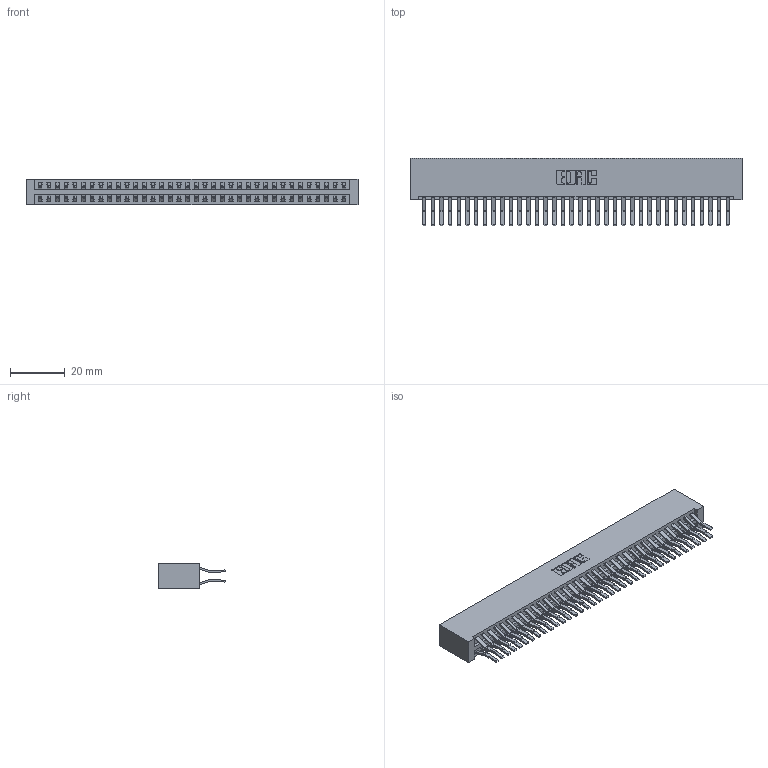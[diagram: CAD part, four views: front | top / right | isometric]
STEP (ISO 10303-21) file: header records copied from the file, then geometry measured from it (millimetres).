
FILE_DESCRIPTION (( 'STEP AP203' ), '1' );
FILE_NAME ('396-072-560-201.STEP', '2018-09-09T11:05:24', ( '' ), ( '' ), 'SwSTEP 2.0', 'SolidWorks 2016', '' );
FILE_SCHEMA (( 'CONFIG_CONTROL_DESIGN' ));
Length unit declared in the file: inch
Products named in the file (3): 346 Part_No Mounting Lugs; 345-292-001_560 Tail; 396-072-560-201
Assembly tree (73 placements, depth 2):
  396-072-560-201
    346 Part_No Mounting Lugs
    345-292-001_560 Tail  x72
Bounding box: 121.54 x 24.78 x 9.4 mm (x, y, z)
Volume: 12850.2 mm3; surface area: 18991.4 mm2
Topology: 73 solids, 73 shells, 4002 faces, 11897 edges, 7834 vertices
Faces by surface type: plane 2592, cylinder 1410
Entity records: 24113 total; most frequent: CARTESIAN_POINT 3980, ORIENTED_EDGE 3914, DIRECTION 3557, EDGE_CURVE 1957, LINE 1685, VECTOR 1685, VERTEX_POINT 1302, AXIS2_PLACEMENT_3D 936
